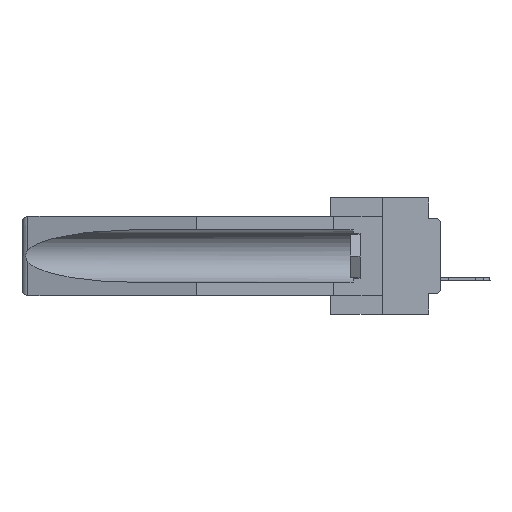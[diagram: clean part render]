
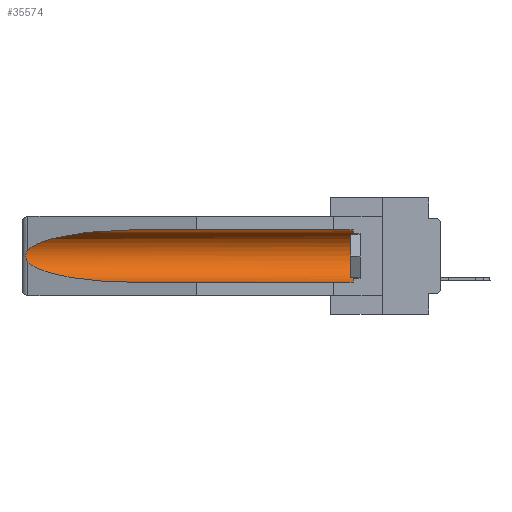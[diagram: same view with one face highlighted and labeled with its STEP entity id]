
A CAD part, left-side view. The second image highlights one B-rep face of the part: STEP entity #35574.
In plain terms, the highlighted cylindrical face has radius 2.857 mm (diameter 5.715 mm), a partial arc.
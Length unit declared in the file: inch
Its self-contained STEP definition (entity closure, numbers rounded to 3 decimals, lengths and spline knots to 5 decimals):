
#50 = DIRECTION ( 'NONE',  ( 0., 1., 0. ) ) ;
#693 = DIRECTION ( 'NONE',  ( 0., 1., 0. ) ) ;
#797 = CARTESIAN_POINT ( 'NONE',  ( 0.26597, 1.5296, -0.19026 ) ) ;
#814 = CARTESIAN_POINT ( 'NONE',  ( 0.155, 1.07973, -0.284 ) ) ;
#1028 = DIRECTION ( 'NONE',  ( 0., 0., 1. ) ) ;
#3395 = DIRECTION ( 'NONE',  ( 0., 0., 1. ) ) ;
#4076 = DIRECTION ( 'NONE',  ( 0., -1., 0. ) ) ;
#4283 = ORIENTED_EDGE ( 'NONE', *, *, #17469, .T. ) ;
#4395 = CARTESIAN_POINT ( 'NONE',  ( 0.155, 0.126, -0.059 ) ) ;
#5350 = VERTEX_POINT ( 'NONE', #4395 ) ;
#5922 = LINE ( 'NONE', #24825, #31384 ) ;
#6111 = ORIENTED_EDGE ( 'NONE', *, *, #12589, .F. ) ;
#6182 = CARTESIAN_POINT ( 'NONE',  ( 0.155, -0.30754, -0.059 ) ) ;
#6216 = CARTESIAN_POINT ( 'NONE',  ( 0.26537, 1.52718, -0.19328 ) ) ;
#6571 = B_SPLINE_CURVE_WITH_KNOTS ( 'NONE', 3,
 ( #20434, #28010, #22573, #14490, #31221, #25457, #30697, #28335, #797, #6216 ),
 .UNSPECIFIED., .F., .F.,
 ( 4, 2, 2, 2, 4 ),
 ( 0., 0.00029, 0.00058, 0.00087, 0.00117 ),
 .UNSPECIFIED. ) ;
#7391 = CARTESIAN_POINT ( 'NONE',  ( 0.26537, 1.52718, -0.14972 ) ) ;
#7536 = CARTESIAN_POINT ( 'NONE',  ( 0.155, 1.07973, -0.284 ) ) ;
#7555 = CARTESIAN_POINT ( 'NONE',  ( 0.155, 0.126, -0.284 ) ) ;
#8903 = VERTEX_POINT ( 'NONE', #7555 ) ;
#9606 = VERTEX_POINT ( 'NONE', #814 ) ;
#10074 = CARTESIAN_POINT ( 'NONE',  ( 0.25451, 1.48313, -0.09465 ) ) ;
#10486 = ORIENTED_EDGE ( 'NONE', *, *, #34633, .T. ) ;
#10888 = VECTOR ( 'NONE', #50, 39.37008 ) ;
#11847 = AXIS2_PLACEMENT_3D ( 'NONE', #25694, #4076, #1028 ) ;
#12314 = AXIS2_PLACEMENT_3D ( 'NONE', #33974, #22985, #3395 ) ;
#12589 = EDGE_CURVE ( 'NONE', #8903, #9606, #5922, .T. ) ;
#12787 = VERTEX_POINT ( 'NONE', #31509 ) ;
#14490 = CARTESIAN_POINT ( 'NONE',  ( 0.2673, 1.5327, -0.16383 ) ) ;
#15480 = CARTESIAN_POINT ( 'NONE',  ( 0.21114, 1.30732, -0.059 ) ) ;
#16019 = CARTESIAN_POINT ( 'NONE',  ( 0.26537, 1.52718, -0.19328 ) ) ;
#17252 = ORIENTED_EDGE ( 'NONE', *, *, #19358, .T. ) ;
#17423 = ORIENTED_EDGE ( 'NONE', *, *, #25837, .T. ) ;
#17469 = EDGE_CURVE ( 'NONE', #12787, #30581, #26224, .T. ) ;
#17481 =( BOUNDED_CURVE ( )  B_SPLINE_CURVE ( 3, ( #16019, #26980, #18493, #7536 ),
 .UNSPECIFIED., .F., .T. ) 
 B_SPLINE_CURVE_WITH_KNOTS ( ( 4, 4 ),
 ( 0.1948, 1.5708 ),
 .UNSPECIFIED. ) 
 CURVE ( )  GEOMETRIC_REPRESENTATION_ITEM ( )  RATIONAL_B_SPLINE_CURVE ( ( 1., 0.848, 0.848, 1. ) ) 
 REPRESENTATION_ITEM ( '' )  );
#18493 = CARTESIAN_POINT ( 'NONE',  ( 0.21114, 1.30732, -0.284 ) ) ;
#18690 = CARTESIAN_POINT ( 'NONE',  ( 0.155, 1.07973, -0.059 ) ) ;
#19358 = EDGE_CURVE ( 'NONE', #30581, #28026, #6571, .T. ) ;
#20434 = CARTESIAN_POINT ( 'NONE',  ( 0.26537, 1.52718, -0.14972 ) ) ;
#22573 = CARTESIAN_POINT ( 'NONE',  ( 0.26654, 1.53092, -0.15636 ) ) ;
#22985 = DIRECTION ( 'NONE',  ( 0., 1., 0. ) ) ;
#24825 = CARTESIAN_POINT ( 'NONE',  ( 0.155, -0.30754, -0.284 ) ) ;
#25457 = CARTESIAN_POINT ( 'NONE',  ( 0.2675, 1.53308, -0.17534 ) ) ;
#25694 = CARTESIAN_POINT ( 'NONE',  ( 0.155, 0.126, -0.1715 ) ) ;
#25837 = EDGE_CURVE ( 'NONE', #28026, #9606, #17481, .T. ) ;
#26094 = EDGE_CURVE ( 'NONE', #8903, #5350, #31380, .T. ) ;
#26224 =( BOUNDED_CURVE ( )  B_SPLINE_CURVE ( 3, ( #18690, #15480, #10074, #26981 ),
 .UNSPECIFIED., .F., .T. ) 
 B_SPLINE_CURVE_WITH_KNOTS ( ( 4, 4 ),
 ( 4.71239, 6.08839 ),
 .UNSPECIFIED. ) 
 CURVE ( )  GEOMETRIC_REPRESENTATION_ITEM ( )  RATIONAL_B_SPLINE_CURVE ( ( 1., 0.848, 0.848, 1. ) ) 
 REPRESENTATION_ITEM ( '' )  );
#26980 = CARTESIAN_POINT ( 'NONE',  ( 0.25451, 1.48313, -0.24835 ) ) ;
#26981 = CARTESIAN_POINT ( 'NONE',  ( 0.26537, 1.52718, -0.14972 ) ) ;
#27725 = CARTESIAN_POINT ( 'NONE',  ( 0.26537, 1.52718, -0.19328 ) ) ;
#27972 = LINE ( 'NONE', #6182, #10888 ) ;
#28010 = CARTESIAN_POINT ( 'NONE',  ( 0.26597, 1.52961, -0.15275 ) ) ;
#28026 = VERTEX_POINT ( 'NONE', #27725 ) ;
#28058 = FACE_OUTER_BOUND ( 'NONE', #30977, .T. ) ;
#28335 = CARTESIAN_POINT ( 'NONE',  ( 0.26655, 1.53094, -0.18657 ) ) ;
#28389 = CYLINDRICAL_SURFACE ( 'NONE', #12314, 0.1125 ) ;
#29158 = ORIENTED_EDGE ( 'NONE', *, *, #26094, .T. ) ;
#30581 = VERTEX_POINT ( 'NONE', #7391 ) ;
#30697 = CARTESIAN_POINT ( 'NONE',  ( 0.2673, 1.53269, -0.17917 ) ) ;
#30977 = EDGE_LOOP ( 'NONE', ( #4283, #17252, #17423, #6111, #29158, #10486 ) ) ;
#31221 = CARTESIAN_POINT ( 'NONE',  ( 0.2675, 1.53308, -0.16763 ) ) ;
#31380 = CIRCLE ( 'NONE', #11847, 0.1125 ) ;
#31384 = VECTOR ( 'NONE', #693, 39.37008 ) ;
#31509 = CARTESIAN_POINT ( 'NONE',  ( 0.155, 1.07973, -0.059 ) ) ;
#33974 = CARTESIAN_POINT ( 'NONE',  ( 0.155, -0.30754, -0.1715 ) ) ;
#34633 = EDGE_CURVE ( 'NONE', #5350, #12787, #27972, .T. ) ;
#35574 = ADVANCED_FACE ( 'NONE', ( #28058 ), #28389, .F. ) ;
